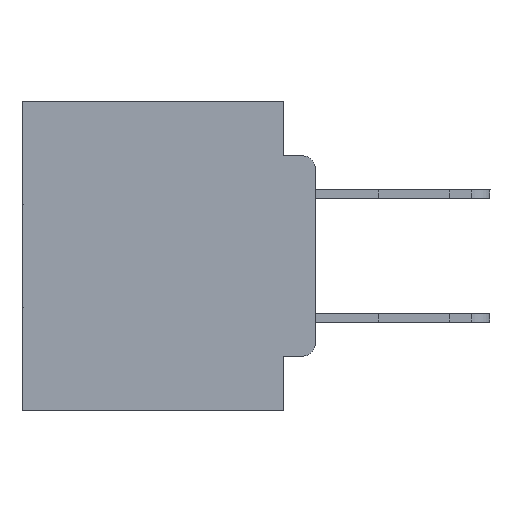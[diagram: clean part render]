
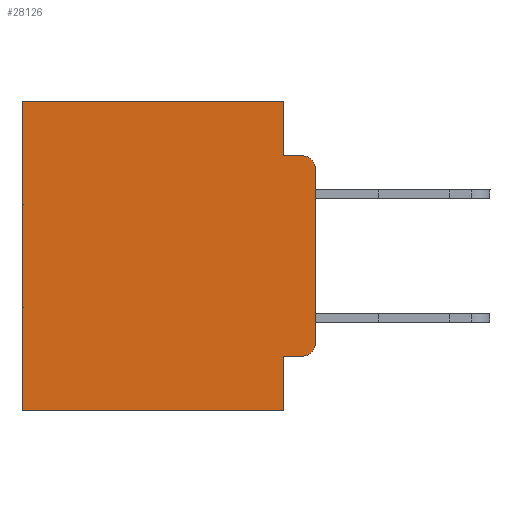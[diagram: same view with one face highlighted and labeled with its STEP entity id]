
A CAD part, left-side view. The second image highlights one B-rep face of the part: STEP entity #28126.
In plain terms, the highlighted planar face has unit normal (-1, 0, 0).
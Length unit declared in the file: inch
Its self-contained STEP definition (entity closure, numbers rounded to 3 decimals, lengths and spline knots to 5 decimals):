
#738 = CIRCLE ( 'NONE', #11989, 0.02 ) ;
#1334 = ORIENTED_EDGE ( 'NONE', *, *, #28753, .T. ) ;
#1789 = LINE ( 'NONE', #15032, #24322 ) ;
#2025 = VECTOR ( 'NONE', #5551, 39.37008 ) ;
#2068 = CARTESIAN_POINT ( 'NONE',  ( 0.298, 0.473, 0. ) ) ;
#2094 = EDGE_CURVE ( 'NONE', #8666, #28054, #27016, .T. ) ;
#2226 = DIRECTION ( 'NONE',  ( 0., 1., 0. ) ) ;
#3348 = CARTESIAN_POINT ( 'NONE',  ( 0.298, 0.473, -0.5 ) ) ;
#5285 = ORIENTED_EDGE ( 'NONE', *, *, #17192, .T. ) ;
#5420 = VERTEX_POINT ( 'NONE', #3348 ) ;
#5551 = DIRECTION ( 'NONE',  ( 0., -1., 0. ) ) ;
#5587 = CARTESIAN_POINT ( 'NONE',  ( 0.298, 0.02, -0.1085 ) ) ;
#5832 = LINE ( 'NONE', #16368, #26598 ) ;
#6284 = VECTOR ( 'NONE', #11613, 39.37008 ) ;
#6288 = EDGE_CURVE ( 'NONE', #22615, #16517, #29680, .T. ) ;
#6328 = DIRECTION ( 'NONE',  ( 0., 0., -1. ) ) ;
#7158 = CARTESIAN_POINT ( 'NONE',  ( 0.298, 0.051, 0. ) ) ;
#7223 = DIRECTION ( 'NONE',  ( -1., 0., 0. ) ) ;
#7307 = CARTESIAN_POINT ( 'NONE',  ( 0.298, 0.02, -0.4115 ) ) ;
#7314 = VERTEX_POINT ( 'NONE', #7307 ) ;
#7530 = LINE ( 'NONE', #21606, #23923 ) ;
#7810 = DIRECTION ( 'NONE',  ( 0., 0., -1. ) ) ;
#7945 = CARTESIAN_POINT ( 'NONE',  ( 0.298, 0.051, -0.5 ) ) ;
#8406 = ORIENTED_EDGE ( 'NONE', *, *, #20795, .T. ) ;
#8666 = VERTEX_POINT ( 'NONE', #24060 ) ;
#10190 = CARTESIAN_POINT ( 'NONE',  ( 0.298, 0.051, 0. ) ) ;
#10225 = CARTESIAN_POINT ( 'NONE',  ( 0.298, 0.051, -0.4115 ) ) ;
#10381 = ORIENTED_EDGE ( 'NONE', *, *, #19334, .F. ) ;
#10992 = ORIENTED_EDGE ( 'NONE', *, *, #18272, .T. ) ;
#11613 = DIRECTION ( 'NONE',  ( 0., 0., -1. ) ) ;
#11739 = ORIENTED_EDGE ( 'NONE', *, *, #24831, .F. ) ;
#11989 = AXIS2_PLACEMENT_3D ( 'NONE', #26159, #7223, #12240 ) ;
#12240 = DIRECTION ( 'NONE',  ( 0., 0., -1. ) ) ;
#12488 = LINE ( 'NONE', #20856, #6284 ) ;
#13030 = EDGE_LOOP ( 'NONE', ( #15373, #16800, #11739, #21711, #10992, #1334, #10381, #16717, #8406, #5285 ) ) ;
#13053 = PLANE ( 'NONE',  #25251 ) ;
#13990 = FACE_OUTER_BOUND ( 'NONE', #13030, .T. ) ;
#14012 = CARTESIAN_POINT ( 'NONE',  ( 0.298, 0.051, -0.0885 ) ) ;
#14128 = VERTEX_POINT ( 'NONE', #27700 ) ;
#14290 = VECTOR ( 'NONE', #29053, 39.37008 ) ;
#14790 = DIRECTION ( 'NONE',  ( 0., 1., 0. ) ) ;
#15032 = CARTESIAN_POINT ( 'NONE',  ( 0.298, 0.051, -0.0885 ) ) ;
#15373 = ORIENTED_EDGE ( 'NONE', *, *, #16534, .F. ) ;
#15493 = DIRECTION ( 'NONE',  ( 1., 0., 0. ) ) ;
#16368 = CARTESIAN_POINT ( 'NONE',  ( 0.298, 0., 0. ) ) ;
#16517 = VERTEX_POINT ( 'NONE', #14012 ) ;
#16534 = EDGE_CURVE ( 'NONE', #22844, #14128, #5832, .T. ) ;
#16717 = ORIENTED_EDGE ( 'NONE', *, *, #2094, .F. ) ;
#16800 = ORIENTED_EDGE ( 'NONE', *, *, #20022, .T. ) ;
#17192 = EDGE_CURVE ( 'NONE', #7314, #14128, #738, .T. ) ;
#18272 = EDGE_CURVE ( 'NONE', #22615, #24341, #21765, .T. ) ;
#19123 = CIRCLE ( 'NONE', #25066, 0.02 ) ;
#19334 = EDGE_CURVE ( 'NONE', #28054, #5420, #7530, .T. ) ;
#20022 = EDGE_CURVE ( 'NONE', #22844, #23611, #19123, .T. ) ;
#20795 = EDGE_CURVE ( 'NONE', #8666, #7314, #27114, .T. ) ;
#20856 = CARTESIAN_POINT ( 'NONE',  ( 0.298, 0.473, 0. ) ) ;
#20862 = CARTESIAN_POINT ( 'NONE',  ( 0.298, 0.051, 0. ) ) ;
#21606 = CARTESIAN_POINT ( 'NONE',  ( 0.298, 0., -0.5 ) ) ;
#21711 = ORIENTED_EDGE ( 'NONE', *, *, #6288, .F. ) ;
#21765 = LINE ( 'NONE', #23166, #22103 ) ;
#22103 = VECTOR ( 'NONE', #2226, 39.37008 ) ;
#22615 = VERTEX_POINT ( 'NONE', #20862 ) ;
#22844 = VERTEX_POINT ( 'NONE', #26424 ) ;
#23166 = CARTESIAN_POINT ( 'NONE',  ( 0.298, 0., 0. ) ) ;
#23611 = VERTEX_POINT ( 'NONE', #23853 ) ;
#23847 = DIRECTION ( 'NONE',  ( 0., 0., -1. ) ) ;
#23853 = CARTESIAN_POINT ( 'NONE',  ( 0.298, 0.02, -0.0885 ) ) ;
#23923 = VECTOR ( 'NONE', #14790, 39.37008 ) ;
#24060 = CARTESIAN_POINT ( 'NONE',  ( 0.298, 0.051, -0.4115 ) ) ;
#24322 = VECTOR ( 'NONE', #26523, 39.37008 ) ;
#24341 = VERTEX_POINT ( 'NONE', #2068 ) ;
#24831 = EDGE_CURVE ( 'NONE', #16517, #23611, #1789, .T. ) ;
#25066 = AXIS2_PLACEMENT_3D ( 'NONE', #5587, #26648, #7810 ) ;
#25251 = AXIS2_PLACEMENT_3D ( 'NONE', #29366, #15493, #6328 ) ;
#25698 = DIRECTION ( 'NONE',  ( 0., 0., -1. ) ) ;
#26159 = CARTESIAN_POINT ( 'NONE',  ( 0.298, 0.02, -0.3915 ) ) ;
#26424 = CARTESIAN_POINT ( 'NONE',  ( 0.298, 0., -0.1085 ) ) ;
#26523 = DIRECTION ( 'NONE',  ( 0., -1., 0. ) ) ;
#26598 = VECTOR ( 'NONE', #25698, 39.37008 ) ;
#26648 = DIRECTION ( 'NONE',  ( -1., 0., 0. ) ) ;
#27016 = LINE ( 'NONE', #10190, #14290 ) ;
#27081 = VECTOR ( 'NONE', #23847, 39.37008 ) ;
#27114 = LINE ( 'NONE', #10225, #2025 ) ;
#27700 = CARTESIAN_POINT ( 'NONE',  ( 0.298, 0., -0.3915 ) ) ;
#28054 = VERTEX_POINT ( 'NONE', #7945 ) ;
#28126 = ADVANCED_FACE ( 'NONE', ( #13990 ), #13053, .F. ) ;
#28753 = EDGE_CURVE ( 'NONE', #24341, #5420, #12488, .T. ) ;
#29053 = DIRECTION ( 'NONE',  ( 0., 0., -1. ) ) ;
#29366 = CARTESIAN_POINT ( 'NONE',  ( 0.298, 0., 0. ) ) ;
#29680 = LINE ( 'NONE', #7158, #27081 ) ;
